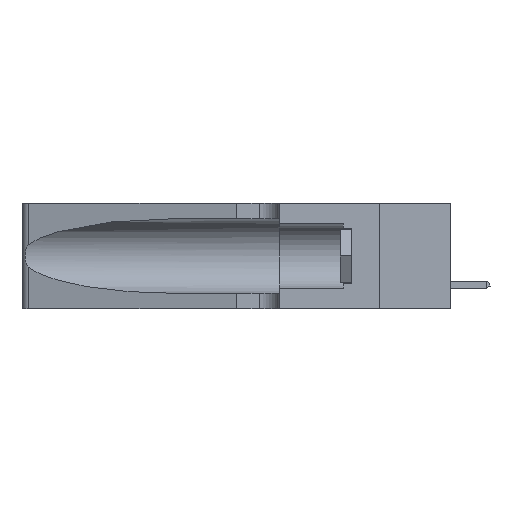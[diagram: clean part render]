
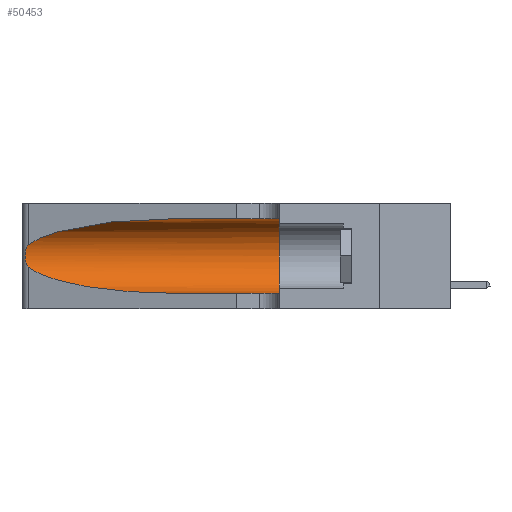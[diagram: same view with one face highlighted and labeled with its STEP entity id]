
A CAD part, left-side view. The second image highlights one B-rep face of the part: STEP entity #50453.
In plain terms, the highlighted cylindrical face has radius 3.308 mm (diameter 6.617 mm), a partial arc.
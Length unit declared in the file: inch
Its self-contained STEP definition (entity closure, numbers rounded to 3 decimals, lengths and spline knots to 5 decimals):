
#248 = VERTEX_POINT ( 'NONE', #50189 ) ;
#1574 = ORIENTED_EDGE ( 'NONE', *, *, #38173, .T. ) ;
#3138 = CARTESIAN_POINT ( 'NONE',  ( 0.2373, 1.15595, 0.28018 ) ) ;
#3678 = LINE ( 'NONE', #45136, #42321 ) ;
#4614 = CARTESIAN_POINT ( 'NONE',  ( 0.25639, 1.23184, 0.21858 ) ) ;
#5004 = VERTEX_POINT ( 'NONE', #44262 ) ;
#5144 = ORIENTED_EDGE ( 'NONE', *, *, #28658, .T. ) ;
#7184 = CARTESIAN_POINT ( 'NONE',  ( 0.25487, 1.22718, 0.22369 ) ) ;
#8057 = CARTESIAN_POINT ( 'NONE',  ( 0.1305, 0.72297, 0.05475 ) ) ;
#8646 = CARTESIAN_POINT ( 'NONE',  ( 0.26018, 1.23835, 0.19895 ) ) ;
#9101 = CARTESIAN_POINT ( 'NONE',  ( 0.25555, 1.22993, 0.14849 ) ) ;
#9441 = CARTESIAN_POINT ( 'NONE',  ( 0.25487, 1.22718, 0.14631 ) ) ;
#9750 = CARTESIAN_POINT ( 'NONE',  ( 0.1305, 0.35, 0.185 ) ) ;
#10915 = LINE ( 'NONE', #49306, #28962 ) ;
#11204 = CARTESIAN_POINT ( 'NONE',  ( 0.18966, 0.96281, 0.31525 ) ) ;
#12715 = CARTESIAN_POINT ( 'NONE',  ( 0.2373, 1.15595, 0.08982 ) ) ;
#12748 = B_SPLINE_CURVE_WITH_KNOTS ( 'NONE', 3,
 ( #27789, #20493, #4614, #40111, #32447, #8646, #28739, #16649, #20651, #20016, #48078, #24077, #9101, #9441 ),
 .UNSPECIFIED., .F., .F.,
 ( 4, 2, 2, 2, 2, 2, 4 ),
 ( 0., 0.00027, 0.00053, 0.00107, 0.0016, 0.00187, 0.00214 ),
 .UNSPECIFIED. ) ;
#13434 = DIRECTION ( 'NONE',  ( 0., -1., 0. ) ) ;
#14063 = CARTESIAN_POINT ( 'NONE',  ( 0.25487, 1.22718, 0.14631 ) ) ;
#15035 = CARTESIAN_POINT ( 'NONE',  ( 0.1305, 0.72297, 0.31525 ) ) ;
#15510 = AXIS2_PLACEMENT_3D ( 'NONE', #44932, #29000, #48948 ) ;
#16290 = CIRCLE ( 'NONE', #34412, 0.13025 ) ;
#16574 = EDGE_CURVE ( 'NONE', #248, #19196, #3678, .T. ) ;
#16649 = CARTESIAN_POINT ( 'NONE',  ( 0.26075, 1.23896, 0.178 ) ) ;
#17602 = CARTESIAN_POINT ( 'NONE',  ( 0.25487, 1.22718, 0.22369 ) ) ;
#17925 = EDGE_CURVE ( 'NONE', #248, #23382, #22664, .T. ) ;
#18138 = DIRECTION ( 'NONE',  ( 0., 0., 1. ) ) ;
#19196 = VERTEX_POINT ( 'NONE', #19462 ) ;
#19393 = EDGE_CURVE ( 'NONE', #23382, #44746, #12748, .T. ) ;
#19462 = CARTESIAN_POINT ( 'NONE',  ( 0.1305, 0.35, 0.31525 ) ) ;
#19562 = CYLINDRICAL_SURFACE ( 'NONE', #15510, 0.13025 ) ;
#20016 = CARTESIAN_POINT ( 'NONE',  ( 0.25856, 1.23593, 0.16098 ) ) ;
#20493 = CARTESIAN_POINT ( 'NONE',  ( 0.25555, 1.22994, 0.2215 ) ) ;
#20651 = CARTESIAN_POINT ( 'NONE',  ( 0.26017, 1.23833, 0.17102 ) ) ;
#22664 =( BOUNDED_CURVE ( )  B_SPLINE_CURVE ( 3, ( #15035, #11204, #3138, #7184 ),
 .UNSPECIFIED., .F., .F. ) 
 B_SPLINE_CURVE_WITH_KNOTS ( ( 4, 4 ),
 ( 1.5708, 2.84003 ),
 .UNSPECIFIED. ) 
 CURVE ( )  GEOMETRIC_REPRESENTATION_ITEM ( )  RATIONAL_B_SPLINE_CURVE ( ( 1., 0.87, 0.87, 1. ) ) 
 REPRESENTATION_ITEM ( '' )  );
#23336 = ORIENTED_EDGE ( 'NONE', *, *, #17925, .T. ) ;
#23382 = VERTEX_POINT ( 'NONE', #17602 ) ;
#24077 = CARTESIAN_POINT ( 'NONE',  ( 0.25639, 1.23186, 0.15144 ) ) ;
#24212 = EDGE_CURVE ( 'NONE', #19196, #25067, #16290, .T. ) ;
#25067 = VERTEX_POINT ( 'NONE', #35448 ) ;
#25334 = DIRECTION ( 'NONE',  ( 0., -1., 0. ) ) ;
#27789 = CARTESIAN_POINT ( 'NONE',  ( 0.25487, 1.22718, 0.22369 ) ) ;
#28658 = EDGE_CURVE ( 'NONE', #5004, #25067, #10915, .T. ) ;
#28739 = CARTESIAN_POINT ( 'NONE',  ( 0.26075, 1.23896, 0.19203 ) ) ;
#28962 = VECTOR ( 'NONE', #13434, 39.37008 ) ;
#29000 = DIRECTION ( 'NONE',  ( 0., -1., 0. ) ) ;
#32447 = CARTESIAN_POINT ( 'NONE',  ( 0.25854, 1.2359, 0.20912 ) ) ;
#34412 = AXIS2_PLACEMENT_3D ( 'NONE', #9750, #49844, #18138 ) ;
#35448 = CARTESIAN_POINT ( 'NONE',  ( 0.1305, 0.35, 0.05475 ) ) ;
#36303 = CARTESIAN_POINT ( 'NONE',  ( 0.25487, 1.22718, 0.14631 ) ) ;
#37333 =( BOUNDED_CURVE ( )  B_SPLINE_CURVE ( 3, ( #36303, #12715, #43792, #8057 ),
 .UNSPECIFIED., .F., .T. ) 
 B_SPLINE_CURVE_WITH_KNOTS ( ( 4, 4 ),
 ( 3.44316, 4.71239 ),
 .UNSPECIFIED. ) 
 CURVE ( )  GEOMETRIC_REPRESENTATION_ITEM ( )  RATIONAL_B_SPLINE_CURVE ( ( 1., 0.87, 0.87, 1. ) ) 
 REPRESENTATION_ITEM ( '' )  );
#38173 = EDGE_CURVE ( 'NONE', #44746, #5004, #37333, .T. ) ;
#38339 = EDGE_LOOP ( 'NONE', ( #23336, #40356, #1574, #5144, #38709, #46040 ) ) ;
#38709 = ORIENTED_EDGE ( 'NONE', *, *, #24212, .F. ) ;
#40111 = CARTESIAN_POINT ( 'NONE',  ( 0.25787, 1.23484, 0.2124 ) ) ;
#40356 = ORIENTED_EDGE ( 'NONE', *, *, #19393, .T. ) ;
#42321 = VECTOR ( 'NONE', #25334, 39.37008 ) ;
#43792 = CARTESIAN_POINT ( 'NONE',  ( 0.18966, 0.96281, 0.05475 ) ) ;
#44262 = CARTESIAN_POINT ( 'NONE',  ( 0.1305, 0.72297, 0.05475 ) ) ;
#44746 = VERTEX_POINT ( 'NONE', #14063 ) ;
#44932 = CARTESIAN_POINT ( 'NONE',  ( 0.1305, 1.61858, 0.185 ) ) ;
#45136 = CARTESIAN_POINT ( 'NONE',  ( 0.1305, 1.61858, 0.31525 ) ) ;
#46040 = ORIENTED_EDGE ( 'NONE', *, *, #16574, .F. ) ;
#48078 = CARTESIAN_POINT ( 'NONE',  ( 0.25789, 1.23486, 0.15765 ) ) ;
#48948 = DIRECTION ( 'NONE',  ( 0., 0., -1. ) ) ;
#49306 = CARTESIAN_POINT ( 'NONE',  ( 0.1305, 1.61858, 0.05475 ) ) ;
#49844 = DIRECTION ( 'NONE',  ( 0., 1., 0. ) ) ;
#50053 = FACE_OUTER_BOUND ( 'NONE', #38339, .T. ) ;
#50189 = CARTESIAN_POINT ( 'NONE',  ( 0.1305, 0.72297, 0.31525 ) ) ;
#50453 = ADVANCED_FACE ( 'NONE', ( #50053 ), #19562, .F. ) ;
